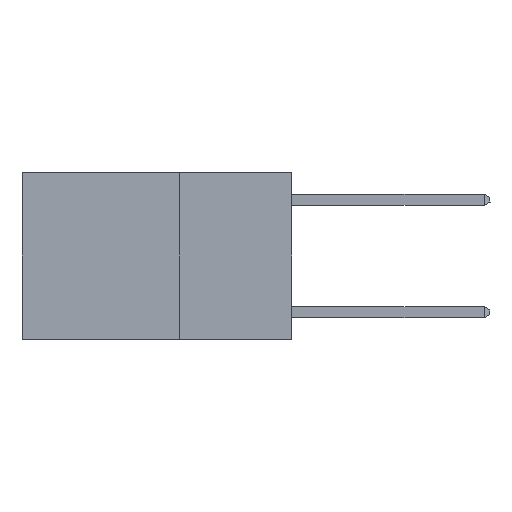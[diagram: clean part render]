
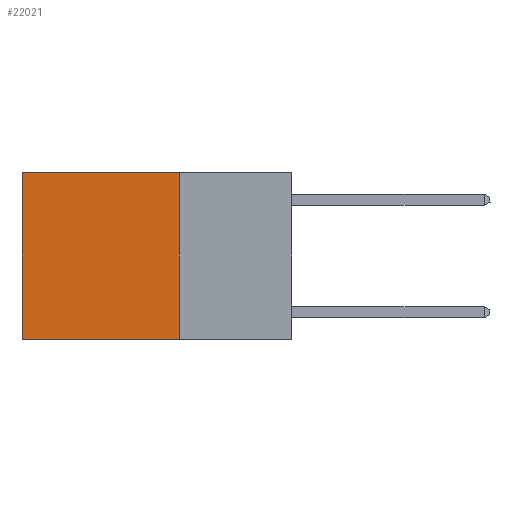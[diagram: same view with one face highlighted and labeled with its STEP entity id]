
A CAD part, left-side view. The second image highlights one B-rep face of the part: STEP entity #22021.
In plain terms, the highlighted planar face has unit normal (-1, 0, 0).
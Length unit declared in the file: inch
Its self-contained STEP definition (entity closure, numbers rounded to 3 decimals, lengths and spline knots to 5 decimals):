
#1528 = CARTESIAN_POINT ( 'NONE',  ( 0.2625, 0.6, 0. ) ) ;
#2893 = DIRECTION ( 'NONE',  ( 0., 0., -1. ) ) ;
#3327 = EDGE_LOOP ( 'NONE', ( #5140, #6330, #17584, #14083 ) ) ;
#3519 = VECTOR ( 'NONE', #17921, 39.37008 ) ;
#4640 = VERTEX_POINT ( 'NONE', #11181 ) ;
#5140 = ORIENTED_EDGE ( 'NONE', *, *, #14406, .T. ) ;
#6330 = ORIENTED_EDGE ( 'NONE', *, *, #19092, .F. ) ;
#7222 = VECTOR ( 'NONE', #7441, 39.37008 ) ;
#7359 = VERTEX_POINT ( 'NONE', #13964 ) ;
#7441 = DIRECTION ( 'NONE',  ( 0., 0., -1. ) ) ;
#7528 = CARTESIAN_POINT ( 'NONE',  ( 0.2625, 0.25, 0. ) ) ;
#7825 = CARTESIAN_POINT ( 'NONE',  ( 0.2625, 0.25, -0.37 ) ) ;
#8378 = EDGE_CURVE ( 'NONE', #7359, #19047, #8991, .T. ) ;
#8991 = LINE ( 'NONE', #17715, #12191 ) ;
#9808 = VECTOR ( 'NONE', #26279, 39.37008 ) ;
#10693 = EDGE_CURVE ( 'NONE', #7359, #19515, #19905, .T. ) ;
#11169 = AXIS2_PLACEMENT_3D ( 'NONE', #15608, #17519, #2893 ) ;
#11181 = CARTESIAN_POINT ( 'NONE',  ( 0.2625, 0.6, -0.37 ) ) ;
#11338 = CARTESIAN_POINT ( 'NONE',  ( 0.2625, 0.25, -0.37 ) ) ;
#11738 = LINE ( 'NONE', #11338, #9808 ) ;
#12191 = VECTOR ( 'NONE', #21717, 39.37008 ) ;
#12444 = CARTESIAN_POINT ( 'NONE',  ( 0.2625, 0.6, 0. ) ) ;
#13964 = CARTESIAN_POINT ( 'NONE',  ( 0.2625, 0.25, 0. ) ) ;
#14083 = ORIENTED_EDGE ( 'NONE', *, *, #8378, .T. ) ;
#14406 = EDGE_CURVE ( 'NONE', #19047, #4640, #20115, .T. ) ;
#14426 = FACE_OUTER_BOUND ( 'NONE', #3327, .T. ) ;
#15608 = CARTESIAN_POINT ( 'NONE',  ( 0.2625, 0.25, 0. ) ) ;
#17519 = DIRECTION ( 'NONE',  ( 1., 0., 0. ) ) ;
#17584 = ORIENTED_EDGE ( 'NONE', *, *, #10693, .F. ) ;
#17715 = CARTESIAN_POINT ( 'NONE',  ( 0.2625, 0.25, 0. ) ) ;
#17921 = DIRECTION ( 'NONE',  ( 0., 0., -1. ) ) ;
#19047 = VERTEX_POINT ( 'NONE', #12444 ) ;
#19092 = EDGE_CURVE ( 'NONE', #19515, #4640, #11738, .T. ) ;
#19515 = VERTEX_POINT ( 'NONE', #7825 ) ;
#19905 = LINE ( 'NONE', #7528, #7222 ) ;
#20115 = LINE ( 'NONE', #1528, #3519 ) ;
#21717 = DIRECTION ( 'NONE',  ( 0., 1., 0. ) ) ;
#22021 = ADVANCED_FACE ( 'NONE', ( #14426 ), #23922, .F. ) ;
#23922 = PLANE ( 'NONE',  #11169 ) ;
#26279 = DIRECTION ( 'NONE',  ( 0., 1., 0. ) ) ;
